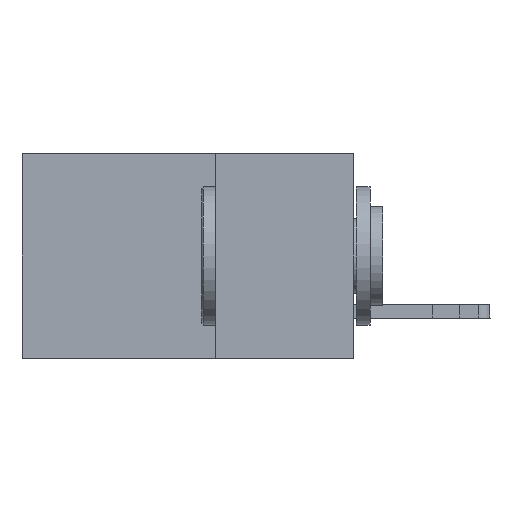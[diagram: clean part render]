
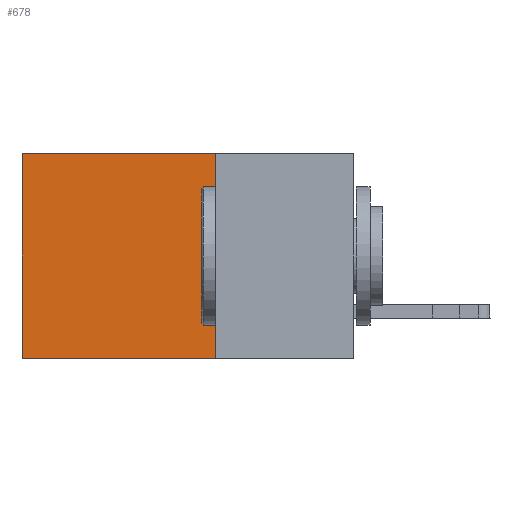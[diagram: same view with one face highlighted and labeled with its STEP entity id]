
A CAD part, left-side view. The second image highlights one B-rep face of the part: STEP entity #678.
In plain terms, the highlighted planar face has unit normal (-1, 0, 0).
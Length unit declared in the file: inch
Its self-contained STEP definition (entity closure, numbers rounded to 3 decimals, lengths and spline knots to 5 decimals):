
#254 = VERTEX_POINT ( 'NONE', #27361 ) ;
#678 = ADVANCED_FACE ( 'NONE', ( #19364 ), #24050, .F. ) ;
#921 = DIRECTION ( 'NONE',  ( 1., 0., 0. ) ) ;
#2509 = VECTOR ( 'NONE', #20075, 39.37008 ) ;
#5619 = CARTESIAN_POINT ( 'NONE',  ( 0.2875, 0.6, 0. ) ) ;
#5770 = CARTESIAN_POINT ( 'NONE',  ( 0.2875, 0.25, 0. ) ) ;
#5851 = EDGE_CURVE ( 'NONE', #13333, #13440, #12409, .T. ) ;
#7328 = CARTESIAN_POINT ( 'NONE',  ( 0.2875, 0.25, 0. ) ) ;
#7666 = LINE ( 'NONE', #7328, #2509 ) ;
#7784 = DIRECTION ( 'NONE',  ( 0., 1., 0. ) ) ;
#7869 = LINE ( 'NONE', #5619, #33947 ) ;
#11279 = DIRECTION ( 'NONE',  ( 0., 0., -1. ) ) ;
#11744 = EDGE_CURVE ( 'NONE', #13440, #27571, #7869, .T. ) ;
#12409 = LINE ( 'NONE', #22931, #33412 ) ;
#12475 = ORIENTED_EDGE ( 'NONE', *, *, #11744, .T. ) ;
#13333 = VERTEX_POINT ( 'NONE', #25615 ) ;
#13440 = VERTEX_POINT ( 'NONE', #18520 ) ;
#13804 = LINE ( 'NONE', #33975, #32478 ) ;
#15912 = ORIENTED_EDGE ( 'NONE', *, *, #19773, .F. ) ;
#18520 = CARTESIAN_POINT ( 'NONE',  ( 0.2875, 0.6, 0. ) ) ;
#19364 = FACE_OUTER_BOUND ( 'NONE', #21021, .T. ) ;
#19773 = EDGE_CURVE ( 'NONE', #13333, #254, #7666, .T. ) ;
#20075 = DIRECTION ( 'NONE',  ( 0., 0., -1. ) ) ;
#20805 = DIRECTION ( 'NONE',  ( 0., 0., -1. ) ) ;
#21021 = EDGE_LOOP ( 'NONE', ( #12475, #25054, #15912, #30389 ) ) ;
#21574 = EDGE_CURVE ( 'NONE', #254, #27571, #13804, .T. ) ;
#22931 = CARTESIAN_POINT ( 'NONE',  ( 0.2875, 0.25, 0. ) ) ;
#23605 = DIRECTION ( 'NONE',  ( 0., 1., 0. ) ) ;
#24050 = PLANE ( 'NONE',  #26127 ) ;
#25054 = ORIENTED_EDGE ( 'NONE', *, *, #21574, .F. ) ;
#25149 = CARTESIAN_POINT ( 'NONE',  ( 0.2875, 0.6, -0.37 ) ) ;
#25615 = CARTESIAN_POINT ( 'NONE',  ( 0.2875, 0.25, 0. ) ) ;
#26127 = AXIS2_PLACEMENT_3D ( 'NONE', #5770, #921, #11279 ) ;
#27361 = CARTESIAN_POINT ( 'NONE',  ( 0.2875, 0.25, -0.37 ) ) ;
#27571 = VERTEX_POINT ( 'NONE', #25149 ) ;
#30389 = ORIENTED_EDGE ( 'NONE', *, *, #5851, .T. ) ;
#32478 = VECTOR ( 'NONE', #7784, 39.37008 ) ;
#33412 = VECTOR ( 'NONE', #23605, 39.37008 ) ;
#33947 = VECTOR ( 'NONE', #20805, 39.37008 ) ;
#33975 = CARTESIAN_POINT ( 'NONE',  ( 0.2875, 0.25, -0.37 ) ) ;
